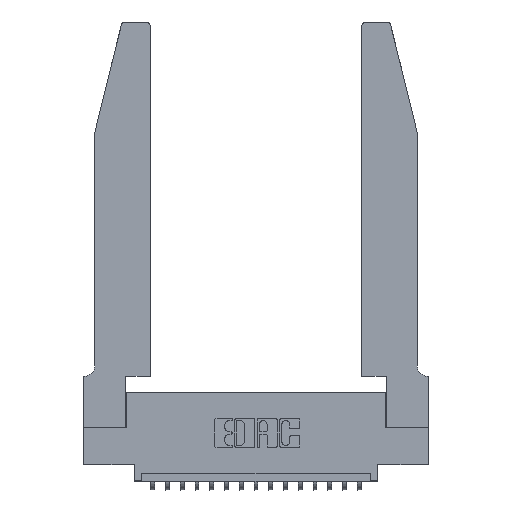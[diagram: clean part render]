
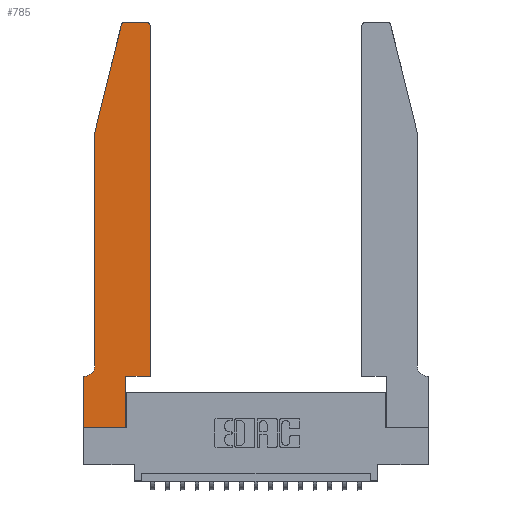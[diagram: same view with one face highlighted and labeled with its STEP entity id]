
A CAD part, top view. The second image highlights one B-rep face of the part: STEP entity #785.
In plain terms, the highlighted planar face has unit normal (0, 0, 1).
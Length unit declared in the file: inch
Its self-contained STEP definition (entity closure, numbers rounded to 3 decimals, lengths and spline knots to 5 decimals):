
#566 = ORIENTED_EDGE ( 'NONE', *, *, #9004, .T. ) ;
#785 = ADVANCED_FACE ( 'NONE', ( #5229 ), #8520, .T. ) ;
#861 = EDGE_CURVE ( 'NONE', #2934, #19856, #16755, .T. ) ;
#920 = VECTOR ( 'NONE', #16548, 39.37008 ) ;
#1056 = VERTEX_POINT ( 'NONE', #18585 ) ;
#1369 = VECTOR ( 'NONE', #19776, 39.37008 ) ;
#1445 = DIRECTION ( 'NONE',  ( 1., 0., 0. ) ) ;
#2362 = ORIENTED_EDGE ( 'NONE', *, *, #13254, .T. ) ;
#2644 = CARTESIAN_POINT ( 'NONE',  ( 0.2865, 0.35, 0.37 ) ) ;
#2722 = VECTOR ( 'NONE', #14576, 39.37008 ) ;
#2731 = AXIS2_PLACEMENT_3D ( 'NONE', #3893, #14479, #11342 ) ;
#2934 = VERTEX_POINT ( 'NONE', #13602 ) ;
#2992 = DIRECTION ( 'NONE',  ( 0., 0., 1. ) ) ;
#3149 = VECTOR ( 'NONE', #12040, 39.37008 ) ;
#3353 = CARTESIAN_POINT ( 'NONE',  ( 0., 0., 0.37 ) ) ;
#3528 = CARTESIAN_POINT ( 'NONE',  ( 0.4505, 2.72, 0.37 ) ) ;
#3777 = ORIENTED_EDGE ( 'NONE', *, *, #9087, .T. ) ;
#3780 = CARTESIAN_POINT ( 'NONE',  ( 0.0755, 2., 0.37 ) ) ;
#3812 = DIRECTION ( 'NONE',  ( 0., 0., -1. ) ) ;
#3893 = CARTESIAN_POINT ( 'NONE',  ( 0., 0.35, 0.37 ) ) ;
#3909 = DIRECTION ( 'NONE',  ( -1., 0., 0. ) ) ;
#4153 = VERTEX_POINT ( 'NONE', #13176 ) ;
#4215 = CARTESIAN_POINT ( 'NONE',  ( 0.0755, 2., 0.37 ) ) ;
#4236 = EDGE_CURVE ( 'NONE', #19856, #4153, #13825, .T. ) ;
#4379 = CARTESIAN_POINT ( 'NONE',  ( 0.284, 2.72, 0.37 ) ) ;
#4589 = VERTEX_POINT ( 'NONE', #3528 ) ;
#4673 = CARTESIAN_POINT ( 'NONE',  ( 0.0755, 2., 0.37 ) ) ;
#4874 = EDGE_CURVE ( 'NONE', #4890, #1056, #17172, .T. ) ;
#4890 = VERTEX_POINT ( 'NONE', #13553 ) ;
#5024 = DIRECTION ( 'NONE',  ( 1., 0., 0. ) ) ;
#5122 = CARTESIAN_POINT ( 'NONE',  ( 0.4205, 2.75, 0.37 ) ) ;
#5124 = LINE ( 'NONE', #5503, #8726 ) ;
#5158 = CARTESIAN_POINT ( 'NONE',  ( 0., 0., 0.37 ) ) ;
#5229 = FACE_OUTER_BOUND ( 'NONE', #17250, .T. ) ;
#5503 = CARTESIAN_POINT ( 'NONE',  ( 0.0755, 0.35, 0.37 ) ) ;
#5705 = CARTESIAN_POINT ( 'NONE',  ( 0., 0.35, 0.37 ) ) ;
#5809 = CARTESIAN_POINT ( 'NONE',  ( 0.0055, 0.35, 0.37 ) ) ;
#5810 = VERTEX_POINT ( 'NONE', #5809 ) ;
#5881 = CARTESIAN_POINT ( 'NONE',  ( 0.4205, 2.72, 0.37 ) ) ;
#6645 = LINE ( 'NONE', #4215, #920 ) ;
#6648 = EDGE_CURVE ( 'NONE', #19676, #4890, #10371, .T. ) ;
#6715 = CARTESIAN_POINT ( 'NONE',  ( 0.4505, 0.35, 0.37 ) ) ;
#7148 = AXIS2_PLACEMENT_3D ( 'NONE', #9839, #3812, #13391 ) ;
#7214 = ORIENTED_EDGE ( 'NONE', *, *, #861, .T. ) ;
#7360 = VECTOR ( 'NONE', #5024, 39.37008 ) ;
#8520 = PLANE ( 'NONE',  #2731 ) ;
#8726 = VECTOR ( 'NONE', #3909, 39.37008 ) ;
#8982 = DIRECTION ( 'NONE',  ( 0., 0., 1. ) ) ;
#9004 = EDGE_CURVE ( 'NONE', #5810, #17755, #5124, .T. ) ;
#9087 = EDGE_CURVE ( 'NONE', #15464, #12104, #16627, .T. ) ;
#9839 = CARTESIAN_POINT ( 'NONE',  ( 0.0055, 0.42, 0.37 ) ) ;
#9947 = DIRECTION ( 'NONE',  ( -1., 0., 0. ) ) ;
#10371 = LINE ( 'NONE', #19099, #13504 ) ;
#11221 = CIRCLE ( 'NONE', #7148, 0.07 ) ;
#11342 = DIRECTION ( 'NONE',  ( 1., 0., 0. ) ) ;
#11373 = AXIS2_PLACEMENT_3D ( 'NONE', #5881, #2992, #16879 ) ;
#11456 = LINE ( 'NONE', #3353, #7360 ) ;
#11655 = LINE ( 'NONE', #6715, #14286 ) ;
#11770 = AXIS2_PLACEMENT_3D ( 'NONE', #4379, #8982, #1445 ) ;
#12040 = DIRECTION ( 'NONE',  ( 0., -1., 0. ) ) ;
#12104 = VERTEX_POINT ( 'NONE', #13115 ) ;
#12645 = CARTESIAN_POINT ( 'NONE',  ( 0., 0., 0.37 ) ) ;
#13071 = CARTESIAN_POINT ( 'NONE',  ( 0.2865, 0.35, 0.37 ) ) ;
#13073 = EDGE_CURVE ( 'NONE', #16935, #2934, #11456, .T. ) ;
#13115 = CARTESIAN_POINT ( 'NONE',  ( 0.0755, 0.42, 0.37 ) ) ;
#13176 = CARTESIAN_POINT ( 'NONE',  ( 0.4505, 0.35, 0.37 ) ) ;
#13254 = EDGE_CURVE ( 'NONE', #1056, #15464, #6645, .T. ) ;
#13391 = DIRECTION ( 'NONE',  ( -1., 0., 0. ) ) ;
#13392 = EDGE_CURVE ( 'NONE', #4589, #19676, #17219, .T. ) ;
#13504 = VECTOR ( 'NONE', #9947, 39.37008 ) ;
#13553 = CARTESIAN_POINT ( 'NONE',  ( 0.284, 2.75, 0.37 ) ) ;
#13602 = CARTESIAN_POINT ( 'NONE',  ( 0.2865, 0., 0.37 ) ) ;
#13706 = ORIENTED_EDGE ( 'NONE', *, *, #15307, .T. ) ;
#13783 = ORIENTED_EDGE ( 'NONE', *, *, #6648, .T. ) ;
#13825 = LINE ( 'NONE', #16870, #1369 ) ;
#14286 = VECTOR ( 'NONE', #14291, 39.37008 ) ;
#14291 = DIRECTION ( 'NONE',  ( 0., 1., 0. ) ) ;
#14479 = DIRECTION ( 'NONE',  ( 0., 0., 1. ) ) ;
#14535 = EDGE_CURVE ( 'NONE', #4153, #4589, #11655, .T. ) ;
#14576 = DIRECTION ( 'NONE',  ( 0., -1., 0. ) ) ;
#14843 = VECTOR ( 'NONE', #16163, 39.37008 ) ;
#15092 = ORIENTED_EDGE ( 'NONE', *, *, #18399, .T. ) ;
#15144 = ORIENTED_EDGE ( 'NONE', *, *, #13073, .T. ) ;
#15307 = EDGE_CURVE ( 'NONE', #17755, #16935, #18749, .T. ) ;
#15464 = VERTEX_POINT ( 'NONE', #4673 ) ;
#16163 = DIRECTION ( 'NONE',  ( 0., 1., 0. ) ) ;
#16236 = ORIENTED_EDGE ( 'NONE', *, *, #14535, .T. ) ;
#16548 = DIRECTION ( 'NONE',  ( -0.239, -0.971, 0. ) ) ;
#16627 = LINE ( 'NONE', #3780, #2722 ) ;
#16755 = LINE ( 'NONE', #13071, #14843 ) ;
#16870 = CARTESIAN_POINT ( 'NONE',  ( 0.4505, 0.35, 0.37 ) ) ;
#16879 = DIRECTION ( 'NONE',  ( 1., 0., 0. ) ) ;
#16935 = VERTEX_POINT ( 'NONE', #12645 ) ;
#17172 = CIRCLE ( 'NONE', #11770, 0.03 ) ;
#17219 = CIRCLE ( 'NONE', #11373, 0.03 ) ;
#17250 = EDGE_LOOP ( 'NONE', ( #13783, #17793, #2362, #3777, #15092, #566, #13706, #15144, #7214, #19774, #16236, #17545 ) ) ;
#17545 = ORIENTED_EDGE ( 'NONE', *, *, #13392, .T. ) ;
#17755 = VERTEX_POINT ( 'NONE', #5705 ) ;
#17793 = ORIENTED_EDGE ( 'NONE', *, *, #4874, .T. ) ;
#18399 = EDGE_CURVE ( 'NONE', #12104, #5810, #11221, .T. ) ;
#18585 = CARTESIAN_POINT ( 'NONE',  ( 0.25487, 2.72718, 0.37 ) ) ;
#18749 = LINE ( 'NONE', #5158, #3149 ) ;
#19099 = CARTESIAN_POINT ( 'NONE',  ( 0.2605, 2.75, 0.37 ) ) ;
#19676 = VERTEX_POINT ( 'NONE', #5122 ) ;
#19774 = ORIENTED_EDGE ( 'NONE', *, *, #4236, .T. ) ;
#19776 = DIRECTION ( 'NONE',  ( 1., 0., 0. ) ) ;
#19856 = VERTEX_POINT ( 'NONE', #2644 ) ;
